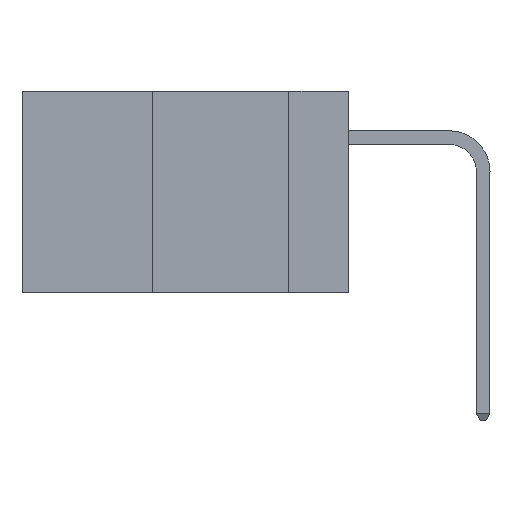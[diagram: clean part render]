
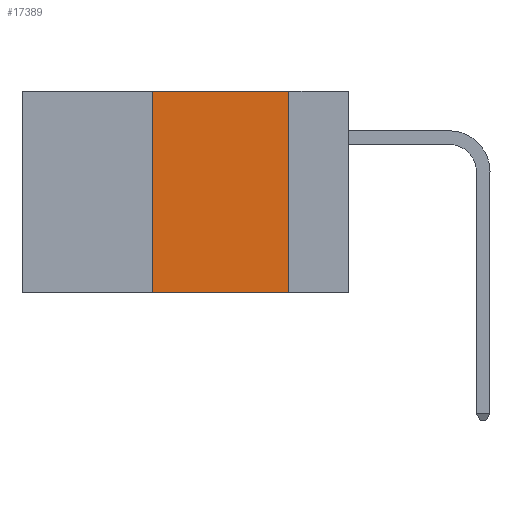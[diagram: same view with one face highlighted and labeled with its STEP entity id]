
A CAD part, left-side view. The second image highlights one B-rep face of the part: STEP entity #17389.
In plain terms, the highlighted planar face has unit normal (-1, 0, 0).
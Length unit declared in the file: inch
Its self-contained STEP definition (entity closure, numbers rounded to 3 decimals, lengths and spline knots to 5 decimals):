
#1487 = CARTESIAN_POINT ( 'NONE',  ( 0., 0.36, 0. ) ) ;
#1685 = AXIS2_PLACEMENT_3D ( 'NONE', #11312, #16088, #21239 ) ;
#2835 = VERTEX_POINT ( 'NONE', #1487 ) ;
#6129 = VERTEX_POINT ( 'NONE', #23793 ) ;
#7723 = ORIENTED_EDGE ( 'NONE', *, *, #31942, .T. ) ;
#10095 = EDGE_LOOP ( 'NONE', ( #28756, #32483, #29862, #7723 ) ) ;
#11312 = CARTESIAN_POINT ( 'NONE',  ( 0., 0.6, 0. ) ) ;
#11329 = FACE_OUTER_BOUND ( 'NONE', #10095, .T. ) ;
#13577 = DIRECTION ( 'NONE',  ( 0., 0., 1. ) ) ;
#14636 = CARTESIAN_POINT ( 'NONE',  ( 0., 0.11, 0. ) ) ;
#15391 = VECTOR ( 'NONE', #13577, 39.37008 ) ;
#16088 = DIRECTION ( 'NONE',  ( 1., 0., 0. ) ) ;
#16314 = VECTOR ( 'NONE', #30720, 39.37008 ) ;
#17389 = ADVANCED_FACE ( 'NONE', ( #11329 ), #21690, .F. ) ;
#17604 = CARTESIAN_POINT ( 'NONE',  ( 0., 0.11, 0. ) ) ;
#20725 = CARTESIAN_POINT ( 'NONE',  ( 0., 0.36, -0.37 ) ) ;
#21205 = CARTESIAN_POINT ( 'NONE',  ( 0., 0.36, 0. ) ) ;
#21239 = DIRECTION ( 'NONE',  ( 0., 0., -1. ) ) ;
#21690 = PLANE ( 'NONE',  #1685 ) ;
#22021 = EDGE_CURVE ( 'NONE', #29663, #6129, #26238, .T. ) ;
#23534 = EDGE_CURVE ( 'NONE', #2835, #29663, #26936, .T. ) ;
#23793 = CARTESIAN_POINT ( 'NONE',  ( 0., 0.11, -0.37 ) ) ;
#24816 = LINE ( 'NONE', #21205, #15391 ) ;
#25014 = VECTOR ( 'NONE', #32904, 39.37008 ) ;
#26238 = LINE ( 'NONE', #14636, #25014 ) ;
#26707 = EDGE_CURVE ( 'NONE', #30889, #2835, #24816, .T. ) ;
#26936 = LINE ( 'NONE', #30962, #16314 ) ;
#27792 = CARTESIAN_POINT ( 'NONE',  ( 0., 0.6, -0.37 ) ) ;
#28756 = ORIENTED_EDGE ( 'NONE', *, *, #22021, .F. ) ;
#29663 = VERTEX_POINT ( 'NONE', #17604 ) ;
#29667 = VECTOR ( 'NONE', #32618, 39.37008 ) ;
#29862 = ORIENTED_EDGE ( 'NONE', *, *, #26707, .F. ) ;
#30720 = DIRECTION ( 'NONE',  ( 0., -1., 0. ) ) ;
#30889 = VERTEX_POINT ( 'NONE', #20725 ) ;
#30962 = CARTESIAN_POINT ( 'NONE',  ( 0., 0.6, 0. ) ) ;
#31942 = EDGE_CURVE ( 'NONE', #30889, #6129, #32951, .T. ) ;
#32483 = ORIENTED_EDGE ( 'NONE', *, *, #23534, .F. ) ;
#32618 = DIRECTION ( 'NONE',  ( 0., -1., 0. ) ) ;
#32904 = DIRECTION ( 'NONE',  ( 0., 0., -1. ) ) ;
#32951 = LINE ( 'NONE', #27792, #29667 ) ;
